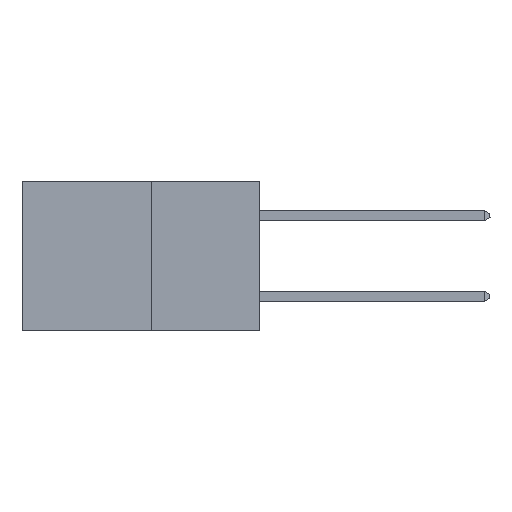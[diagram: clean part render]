
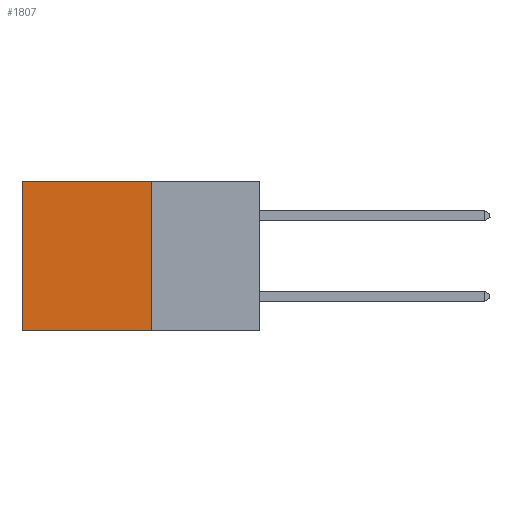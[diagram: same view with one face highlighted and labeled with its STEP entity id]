
A CAD part, left-side view. The second image highlights one B-rep face of the part: STEP entity #1807.
In plain terms, the highlighted planar face has unit normal (-1, 0, 0).
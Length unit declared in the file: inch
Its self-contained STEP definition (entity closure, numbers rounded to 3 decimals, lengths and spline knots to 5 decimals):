
#475 = CARTESIAN_POINT ( 'NONE',  ( 0.277, 0.59, -0.37 ) ) ;
#1715 = LINE ( 'NONE', #12766, #18409 ) ;
#1807 = ADVANCED_FACE ( 'NONE', ( #7145 ), #4366, .F. ) ;
#2410 = ORIENTED_EDGE ( 'NONE', *, *, #17713, .F. ) ;
#3186 = DIRECTION ( 'NONE',  ( 0., 0., -1. ) ) ;
#3449 = CARTESIAN_POINT ( 'NONE',  ( 0.277, 0.27, -0.37 ) ) ;
#4366 = PLANE ( 'NONE',  #17554 ) ;
#4841 = DIRECTION ( 'NONE',  ( 0., 0., -1. ) ) ;
#5749 = VECTOR ( 'NONE', #18110, 39.37008 ) ;
#6161 = EDGE_LOOP ( 'NONE', ( #10904, #17121, #2410, #11667 ) ) ;
#6978 = VERTEX_POINT ( 'NONE', #3449 ) ;
#6980 = CARTESIAN_POINT ( 'NONE',  ( 0.277, 0.27, -0.37 ) ) ;
#7145 = FACE_OUTER_BOUND ( 'NONE', #6161, .T. ) ;
#7228 = EDGE_CURVE ( 'NONE', #6978, #15175, #8323, .T. ) ;
#8323 = LINE ( 'NONE', #14912, #12459 ) ;
#8345 = DIRECTION ( 'NONE',  ( 1., 0., 0. ) ) ;
#8426 = VECTOR ( 'NONE', #15788, 39.37008 ) ;
#10904 = ORIENTED_EDGE ( 'NONE', *, *, #12039, .T. ) ;
#11020 = CARTESIAN_POINT ( 'NONE',  ( 0.277, 0.59, 0. ) ) ;
#11667 = ORIENTED_EDGE ( 'NONE', *, *, #14209, .T. ) ;
#12039 = EDGE_CURVE ( 'NONE', #16184, #15175, #14010, .T. ) ;
#12459 = VECTOR ( 'NONE', #15580, 39.37008 ) ;
#12766 = CARTESIAN_POINT ( 'NONE',  ( 0.277, 0.27, -0.37 ) ) ;
#13059 = CARTESIAN_POINT ( 'NONE',  ( 0.277, 0.59, -0.37 ) ) ;
#14010 = LINE ( 'NONE', #475, #5749 ) ;
#14209 = EDGE_CURVE ( 'NONE', #18102, #16184, #16576, .T. ) ;
#14912 = CARTESIAN_POINT ( 'NONE',  ( 0.277, 0.27, -0.37 ) ) ;
#15175 = VERTEX_POINT ( 'NONE', #13059 ) ;
#15580 = DIRECTION ( 'NONE',  ( 0., 1., 0. ) ) ;
#15788 = DIRECTION ( 'NONE',  ( 0., 1., 0. ) ) ;
#16184 = VERTEX_POINT ( 'NONE', #11020 ) ;
#16576 = LINE ( 'NONE', #17244, #8426 ) ;
#16595 = CARTESIAN_POINT ( 'NONE',  ( 0.277, 0.27, 0. ) ) ;
#17121 = ORIENTED_EDGE ( 'NONE', *, *, #7228, .F. ) ;
#17244 = CARTESIAN_POINT ( 'NONE',  ( 0.277, 0.27, 0. ) ) ;
#17554 = AXIS2_PLACEMENT_3D ( 'NONE', #6980, #8345, #4841 ) ;
#17713 = EDGE_CURVE ( 'NONE', #18102, #6978, #1715, .T. ) ;
#18102 = VERTEX_POINT ( 'NONE', #16595 ) ;
#18110 = DIRECTION ( 'NONE',  ( 0., 0., -1. ) ) ;
#18409 = VECTOR ( 'NONE', #3186, 39.37008 ) ;
